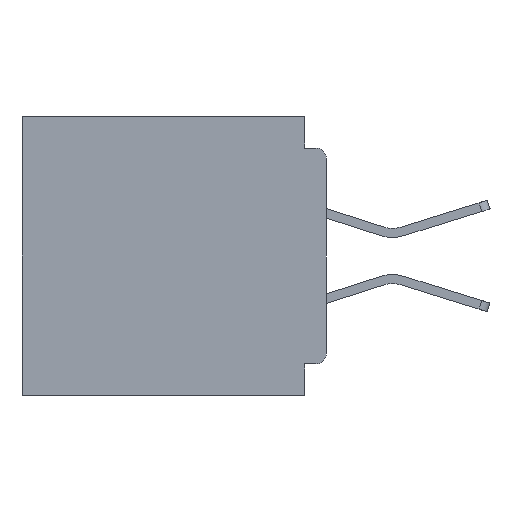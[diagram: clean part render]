
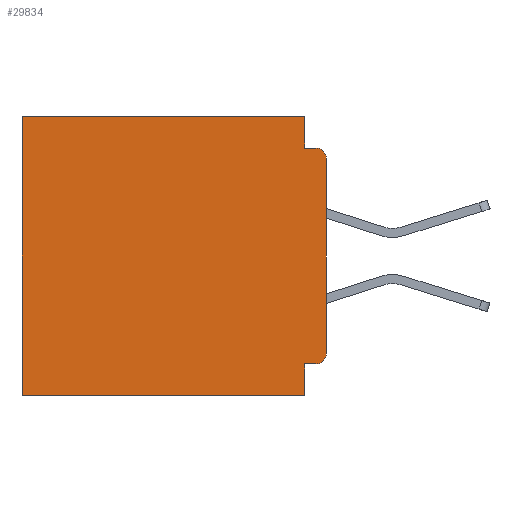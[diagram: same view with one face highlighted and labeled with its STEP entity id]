
A CAD part, left-side view. The second image highlights one B-rep face of the part: STEP entity #29834.
In plain terms, the highlighted planar face has unit normal (-1, 0, 0).
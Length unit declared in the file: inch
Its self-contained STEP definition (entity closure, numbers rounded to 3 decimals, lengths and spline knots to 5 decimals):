
#62 = AXIS2_PLACEMENT_3D ( 'NONE', #12525, #3546, #24591 ) ;
#882 = VECTOR ( 'NONE', #24552, 39.37008 ) ;
#1086 = LINE ( 'NONE', #35561, #32106 ) ;
#1332 = VERTEX_POINT ( 'NONE', #4085 ) ;
#1719 = ORIENTED_EDGE ( 'NONE', *, *, #27889, .F. ) ;
#2376 = CARTESIAN_POINT ( 'NONE',  ( 0.3, 0., -0.355 ) ) ;
#2639 = CARTESIAN_POINT ( 'NONE',  ( 0.3, 0.015, -0.355 ) ) ;
#3434 = VECTOR ( 'NONE', #27995, 39.37008 ) ;
#3546 = DIRECTION ( 'NONE',  ( 1., 0., 0. ) ) ;
#4085 = CARTESIAN_POINT ( 'NONE',  ( 0.3, 0.031, -0.045 ) ) ;
#4240 = EDGE_CURVE ( 'NONE', #38608, #19852, #24859, .T. ) ;
#5353 = DIRECTION ( 'NONE',  ( 0., 1., 0. ) ) ;
#6005 = CARTESIAN_POINT ( 'NONE',  ( 0.3, 0.031, 0. ) ) ;
#7255 = CARTESIAN_POINT ( 'NONE',  ( 0.3, 0.437, -0.4 ) ) ;
#7452 = CARTESIAN_POINT ( 'NONE',  ( 0.3, 0.015, -0.045 ) ) ;
#8084 = EDGE_CURVE ( 'NONE', #19852, #22869, #34467, .T. ) ;
#8197 = VERTEX_POINT ( 'NONE', #7452 ) ;
#8314 = VERTEX_POINT ( 'NONE', #28905 ) ;
#8839 = ORIENTED_EDGE ( 'NONE', *, *, #17497, .F. ) ;
#8973 = EDGE_CURVE ( 'NONE', #33258, #16616, #1086, .T. ) ;
#10005 = CIRCLE ( 'NONE', #24107, 0.015 ) ;
#10801 = EDGE_CURVE ( 'NONE', #16616, #22869, #28709, .T. ) ;
#11958 = DIRECTION ( 'NONE',  ( -1., 0., 0. ) ) ;
#12159 = ORIENTED_EDGE ( 'NONE', *, *, #8973, .F. ) ;
#12525 = CARTESIAN_POINT ( 'NONE',  ( 0.3, 0., -0.4 ) ) ;
#12926 = VECTOR ( 'NONE', #5353, 39.37008 ) ;
#12988 = CARTESIAN_POINT ( 'NONE',  ( 0.3, 0.031, -0.4 ) ) ;
#13066 = CARTESIAN_POINT ( 'NONE',  ( 0.3, 0.437, -0.4 ) ) ;
#13094 = DIRECTION ( 'NONE',  ( 0., 0., -1. ) ) ;
#13233 = CARTESIAN_POINT ( 'NONE',  ( 0.3, 0.437, 0. ) ) ;
#14059 = CARTESIAN_POINT ( 'NONE',  ( 0.3, 0.031, -0.355 ) ) ;
#14393 = CIRCLE ( 'NONE', #21076, 0.015 ) ;
#14451 = ORIENTED_EDGE ( 'NONE', *, *, #4240, .T. ) ;
#14693 = EDGE_CURVE ( 'NONE', #36524, #8314, #24172, .T. ) ;
#15034 = VERTEX_POINT ( 'NONE', #2639 ) ;
#15596 = VECTOR ( 'NONE', #34223, 39.37008 ) ;
#16383 = ORIENTED_EDGE ( 'NONE', *, *, #10801, .F. ) ;
#16415 = DIRECTION ( 'NONE',  ( 0., 0., -1. ) ) ;
#16616 = VERTEX_POINT ( 'NONE', #12988 ) ;
#16760 = ORIENTED_EDGE ( 'NONE', *, *, #14693, .F. ) ;
#17497 = EDGE_CURVE ( 'NONE', #15034, #33258, #36846, .T. ) ;
#17970 = DIRECTION ( 'NONE',  ( -1., 0., 0. ) ) ;
#18227 = ORIENTED_EDGE ( 'NONE', *, *, #8084, .T. ) ;
#18513 = CARTESIAN_POINT ( 'NONE',  ( 0.3, 0.031, 0. ) ) ;
#19827 = EDGE_CURVE ( 'NONE', #1332, #8197, #23584, .T. ) ;
#19852 = VERTEX_POINT ( 'NONE', #13233 ) ;
#20355 = VECTOR ( 'NONE', #13094, 39.37008 ) ;
#20743 = VECTOR ( 'NONE', #28172, 39.37008 ) ;
#21076 = AXIS2_PLACEMENT_3D ( 'NONE', #35941, #17970, #16415 ) ;
#21442 = EDGE_CURVE ( 'NONE', #15034, #8314, #14393, .T. ) ;
#21455 = ORIENTED_EDGE ( 'NONE', *, *, #22562, .T. ) ;
#22562 = EDGE_CURVE ( 'NONE', #36524, #8197, #10005, .T. ) ;
#22869 = VERTEX_POINT ( 'NONE', #7255 ) ;
#23584 = LINE ( 'NONE', #25166, #15596 ) ;
#24107 = AXIS2_PLACEMENT_3D ( 'NONE', #29926, #11958, #32937 ) ;
#24172 = LINE ( 'NONE', #28024, #20355 ) ;
#24552 = DIRECTION ( 'NONE',  ( 0., 1., 0. ) ) ;
#24591 = DIRECTION ( 'NONE',  ( 0., 0., -1. ) ) ;
#24601 = CARTESIAN_POINT ( 'NONE',  ( 0.3, 0., 0. ) ) ;
#24770 = FACE_OUTER_BOUND ( 'NONE', #35082, .T. ) ;
#24859 = LINE ( 'NONE', #24601, #882 ) ;
#25166 = CARTESIAN_POINT ( 'NONE',  ( 0.3, 0., -0.045 ) ) ;
#26624 = DIRECTION ( 'NONE',  ( 0., 0., -1. ) ) ;
#27889 = EDGE_CURVE ( 'NONE', #38608, #1332, #37573, .T. ) ;
#27995 = DIRECTION ( 'NONE',  ( 0., 0., -1. ) ) ;
#28024 = CARTESIAN_POINT ( 'NONE',  ( 0.3, 0., -0.4 ) ) ;
#28172 = DIRECTION ( 'NONE',  ( 0., 1., 0. ) ) ;
#28709 = LINE ( 'NONE', #34084, #20743 ) ;
#28905 = CARTESIAN_POINT ( 'NONE',  ( 0.3, 0., -0.34 ) ) ;
#29621 = VECTOR ( 'NONE', #32985, 39.37008 ) ;
#29834 = ADVANCED_FACE ( 'NONE', ( #24770 ), #33511, .F. ) ;
#29926 = CARTESIAN_POINT ( 'NONE',  ( 0.3, 0.015, -0.06 ) ) ;
#31326 = ORIENTED_EDGE ( 'NONE', *, *, #19827, .F. ) ;
#32106 = VECTOR ( 'NONE', #26624, 39.37008 ) ;
#32316 = CARTESIAN_POINT ( 'NONE',  ( 0.3, 0., -0.06 ) ) ;
#32826 = ORIENTED_EDGE ( 'NONE', *, *, #21442, .T. ) ;
#32937 = DIRECTION ( 'NONE',  ( 0., 0., -1. ) ) ;
#32985 = DIRECTION ( 'NONE',  ( 0., 0., -1. ) ) ;
#33258 = VERTEX_POINT ( 'NONE', #14059 ) ;
#33511 = PLANE ( 'NONE',  #62 ) ;
#34084 = CARTESIAN_POINT ( 'NONE',  ( 0.3, 0., -0.4 ) ) ;
#34223 = DIRECTION ( 'NONE',  ( 0., -1., 0. ) ) ;
#34467 = LINE ( 'NONE', #13066, #3434 ) ;
#35082 = EDGE_LOOP ( 'NONE', ( #16760, #21455, #31326, #1719, #14451, #18227, #16383, #12159, #8839, #32826 ) ) ;
#35561 = CARTESIAN_POINT ( 'NONE',  ( 0.3, 0.031, -0.4 ) ) ;
#35941 = CARTESIAN_POINT ( 'NONE',  ( 0.3, 0.015, -0.34 ) ) ;
#36524 = VERTEX_POINT ( 'NONE', #32316 ) ;
#36846 = LINE ( 'NONE', #2376, #12926 ) ;
#37573 = LINE ( 'NONE', #6005, #29621 ) ;
#38608 = VERTEX_POINT ( 'NONE', #18513 ) ;
